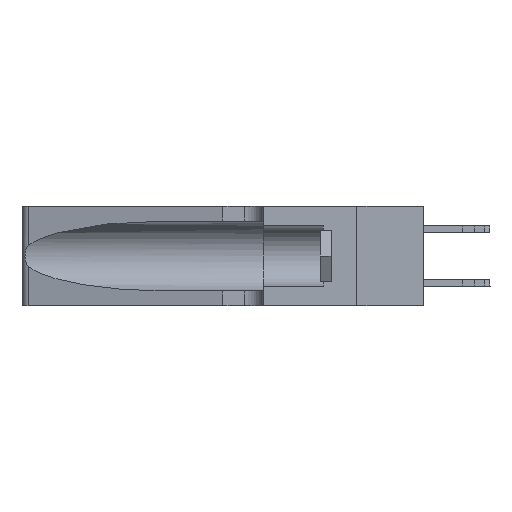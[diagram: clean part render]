
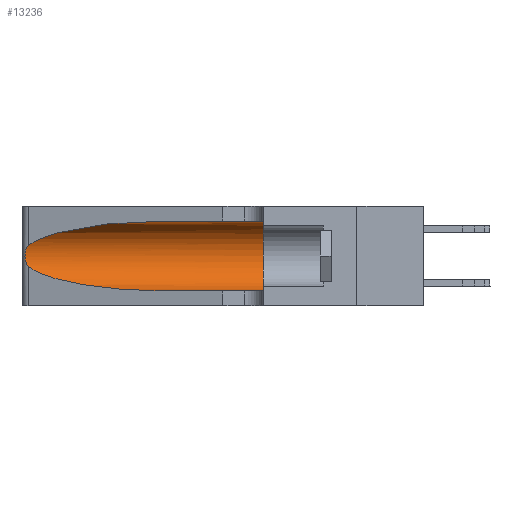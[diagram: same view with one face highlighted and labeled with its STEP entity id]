
A CAD part, left-side view. The second image highlights one B-rep face of the part: STEP entity #13236.
In plain terms, the highlighted cylindrical face has radius 3.308 mm (diameter 6.617 mm), a partial arc.
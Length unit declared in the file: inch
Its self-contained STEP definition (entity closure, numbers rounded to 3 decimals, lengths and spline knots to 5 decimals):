
#120 = CARTESIAN_POINT ( 'NONE',  ( 0.26075, 1.23896, 0.19203 ) ) ;
#212 = CARTESIAN_POINT ( 'NONE',  ( 0.25789, 1.23486, 0.15765 ) ) ;
#408 = ORIENTED_EDGE ( 'NONE', *, *, #11529, .T. ) ;
#789 = EDGE_CURVE ( 'NONE', #2751, #8364, #20169, .T. ) ;
#1045 = CARTESIAN_POINT ( 'NONE',  ( 0.1305, 0.72297, 0.31525 ) ) ;
#1134 = CARTESIAN_POINT ( 'NONE',  ( 0.1305, 0.72297, 0.05475 ) ) ;
#1180 = CARTESIAN_POINT ( 'NONE',  ( 0.1305, 0.72297, 0.05475 ) ) ;
#1804 = DIRECTION ( 'NONE',  ( 0., -1., 0. ) ) ;
#2501 = CARTESIAN_POINT ( 'NONE',  ( 0.25487, 1.22718, 0.14631 ) ) ;
#2599 = CARTESIAN_POINT ( 'NONE',  ( 0.26017, 1.23833, 0.17102 ) ) ;
#2714 = CARTESIAN_POINT ( 'NONE',  ( 0.25854, 1.2359, 0.20912 ) ) ;
#2751 = VERTEX_POINT ( 'NONE', #29762 ) ;
#6165 = EDGE_LOOP ( 'NONE', ( #408, #16625, #20147, #18981, #6595, #16956 ) ) ;
#6411 = CARTESIAN_POINT ( 'NONE',  ( 0.25487, 1.22718, 0.22369 ) ) ;
#6595 = ORIENTED_EDGE ( 'NONE', *, *, #12639, .F. ) ;
#6659 = CARTESIAN_POINT ( 'NONE',  ( 0.1305, 0.35, 0.05475 ) ) ;
#7654 = CYLINDRICAL_SURFACE ( 'NONE', #10667, 0.13025 ) ;
#8003 = DIRECTION ( 'NONE',  ( 0., 1., 0. ) ) ;
#8364 = VERTEX_POINT ( 'NONE', #1134 ) ;
#9026 = VECTOR ( 'NONE', #14215, 39.37008 ) ;
#9368 = CARTESIAN_POINT ( 'NONE',  ( 0.25487, 1.22718, 0.14631 ) ) ;
#9719 = CIRCLE ( 'NONE', #25787, 0.13025 ) ;
#10398 = CARTESIAN_POINT ( 'NONE',  ( 0.25555, 1.22993, 0.14849 ) ) ;
#10505 = CARTESIAN_POINT ( 'NONE',  ( 0.25487, 1.22718, 0.22369 ) ) ;
#10663 = DIRECTION ( 'NONE',  ( 0., 0., 1. ) ) ;
#10667 = AXIS2_PLACEMENT_3D ( 'NONE', #26289, #15233, #31284 ) ;
#10795 = LINE ( 'NONE', #34050, #30318 ) ;
#11445 = CARTESIAN_POINT ( 'NONE',  ( 0.1305, 1.61858, 0.31525 ) ) ;
#11529 = EDGE_CURVE ( 'NONE', #24517, #20914, #30132, .T. ) ;
#12404 = CARTESIAN_POINT ( 'NONE',  ( 0.2373, 1.15595, 0.08982 ) ) ;
#12639 = EDGE_CURVE ( 'NONE', #15747, #13996, #9719, .T. ) ;
#13236 = ADVANCED_FACE ( 'NONE', ( #29244 ), #7654, .F. ) ;
#13367 = CARTESIAN_POINT ( 'NONE',  ( 0.25639, 1.23186, 0.15144 ) ) ;
#13470 = CARTESIAN_POINT ( 'NONE',  ( 0.25856, 1.23593, 0.16098 ) ) ;
#13996 = VERTEX_POINT ( 'NONE', #6659 ) ;
#14215 = DIRECTION ( 'NONE',  ( 0., -1., 0. ) ) ;
#15233 = DIRECTION ( 'NONE',  ( 0., -1., 0. ) ) ;
#15747 = VERTEX_POINT ( 'NONE', #25097 ) ;
#16129 = LINE ( 'NONE', #11445, #9026 ) ;
#16625 = ORIENTED_EDGE ( 'NONE', *, *, #28632, .T. ) ;
#16956 = ORIENTED_EDGE ( 'NONE', *, *, #24852, .F. ) ;
#17506 = CARTESIAN_POINT ( 'NONE',  ( 0.18966, 0.96281, 0.05475 ) ) ;
#18981 = ORIENTED_EDGE ( 'NONE', *, *, #23883, .T. ) ;
#20147 = ORIENTED_EDGE ( 'NONE', *, *, #789, .T. ) ;
#20169 =( BOUNDED_CURVE ( )  B_SPLINE_CURVE ( 3, ( #9368, #12404, #17506, #1180 ),
 .UNSPECIFIED., .F., .F. ) 
 B_SPLINE_CURVE_WITH_KNOTS ( ( 4, 4 ),
 ( 3.44316, 4.71239 ),
 .UNSPECIFIED. ) 
 CURVE ( )  GEOMETRIC_REPRESENTATION_ITEM ( )  RATIONAL_B_SPLINE_CURVE ( ( 1., 0.87, 0.87, 1. ) ) 
 REPRESENTATION_ITEM ( '' )  );
#20914 = VERTEX_POINT ( 'NONE', #6411 ) ;
#21212 = CARTESIAN_POINT ( 'NONE',  ( 0.1305, 0.35, 0.185 ) ) ;
#21379 = CARTESIAN_POINT ( 'NONE',  ( 0.26075, 1.23896, 0.178 ) ) ;
#23883 = EDGE_CURVE ( 'NONE', #8364, #13996, #10795, .T. ) ;
#24517 = VERTEX_POINT ( 'NONE', #32748 ) ;
#24852 = EDGE_CURVE ( 'NONE', #24517, #15747, #16129, .T. ) ;
#24943 = CARTESIAN_POINT ( 'NONE',  ( 0.25487, 1.22718, 0.22369 ) ) ;
#25063 = CARTESIAN_POINT ( 'NONE',  ( 0.2373, 1.15595, 0.28018 ) ) ;
#25097 = CARTESIAN_POINT ( 'NONE',  ( 0.1305, 0.35, 0.31525 ) ) ;
#25787 = AXIS2_PLACEMENT_3D ( 'NONE', #21212, #8003, #10663 ) ;
#26289 = CARTESIAN_POINT ( 'NONE',  ( 0.1305, 1.61858, 0.185 ) ) ;
#28632 = EDGE_CURVE ( 'NONE', #20914, #2751, #32124, .T. ) ;
#29196 = CARTESIAN_POINT ( 'NONE',  ( 0.25787, 1.23484, 0.2124 ) ) ;
#29244 = FACE_OUTER_BOUND ( 'NONE', #6165, .T. ) ;
#29306 = CARTESIAN_POINT ( 'NONE',  ( 0.25639, 1.23184, 0.21858 ) ) ;
#29408 = CARTESIAN_POINT ( 'NONE',  ( 0.25555, 1.22994, 0.2215 ) ) ;
#29762 = CARTESIAN_POINT ( 'NONE',  ( 0.25487, 1.22718, 0.14631 ) ) ;
#30132 =( BOUNDED_CURVE ( )  B_SPLINE_CURVE ( 3, ( #1045, #32709, #25063, #24943 ),
 .UNSPECIFIED., .F., .F. ) 
 B_SPLINE_CURVE_WITH_KNOTS ( ( 4, 4 ),
 ( 1.5708, 2.84003 ),
 .UNSPECIFIED. ) 
 CURVE ( )  GEOMETRIC_REPRESENTATION_ITEM ( )  RATIONAL_B_SPLINE_CURVE ( ( 1., 0.87, 0.87, 1. ) ) 
 REPRESENTATION_ITEM ( '' )  );
#30318 = VECTOR ( 'NONE', #1804, 39.37008 ) ;
#31284 = DIRECTION ( 'NONE',  ( 0., 0., -1. ) ) ;
#31776 = CARTESIAN_POINT ( 'NONE',  ( 0.26018, 1.23835, 0.19895 ) ) ;
#32124 = B_SPLINE_CURVE_WITH_KNOTS ( 'NONE', 3,
 ( #10505, #29408, #29306, #29196, #2714, #31776, #120, #21379, #2599, #13470, #212, #13367, #10398, #2501 ),
 .UNSPECIFIED., .F., .F.,
 ( 4, 2, 2, 2, 2, 2, 4 ),
 ( 0., 0.00027, 0.00053, 0.00107, 0.0016, 0.00187, 0.00214 ),
 .UNSPECIFIED. ) ;
#32709 = CARTESIAN_POINT ( 'NONE',  ( 0.18966, 0.96281, 0.31525 ) ) ;
#32748 = CARTESIAN_POINT ( 'NONE',  ( 0.1305, 0.72297, 0.31525 ) ) ;
#34050 = CARTESIAN_POINT ( 'NONE',  ( 0.1305, 1.61858, 0.05475 ) ) ;
